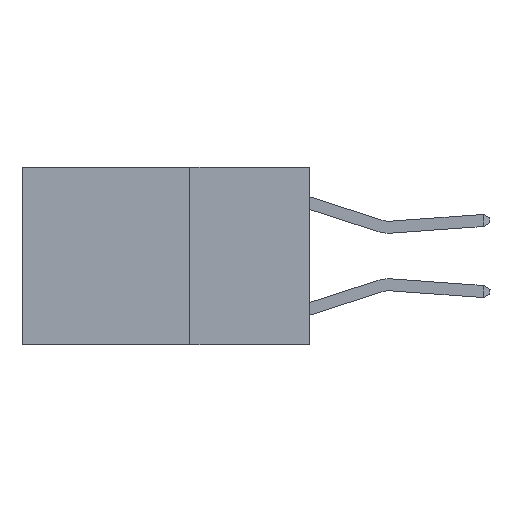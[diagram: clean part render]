
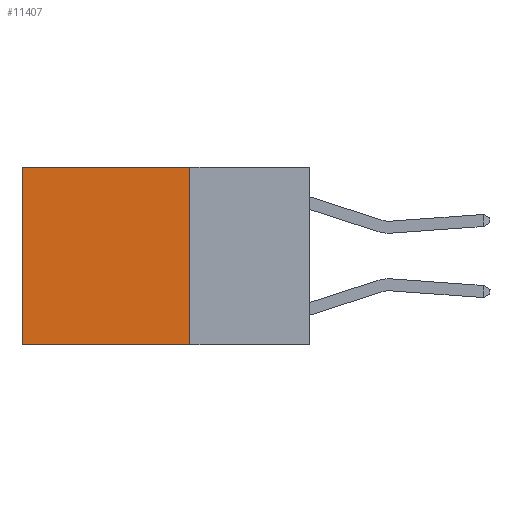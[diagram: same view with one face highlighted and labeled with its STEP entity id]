
A CAD part, left-side view. The second image highlights one B-rep face of the part: STEP entity #11407.
In plain terms, the highlighted planar face has unit normal (-1, 0, 0).
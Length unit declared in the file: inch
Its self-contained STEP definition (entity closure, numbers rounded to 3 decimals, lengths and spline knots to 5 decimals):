
#287 = CARTESIAN_POINT ( 'NONE',  ( 0.2625, 0.6, 0. ) ) ;
#1369 = DIRECTION ( 'NONE',  ( 0., 1., 0. ) ) ;
#1651 = VERTEX_POINT ( 'NONE', #30114 ) ;
#2942 = CARTESIAN_POINT ( 'NONE',  ( 0.2625, 0.25, -0.37 ) ) ;
#3785 = VECTOR ( 'NONE', #29052, 39.37008 ) ;
#3902 = DIRECTION ( 'NONE',  ( 1., 0., 0. ) ) ;
#5384 = ORIENTED_EDGE ( 'NONE', *, *, #7883, .T. ) ;
#6735 = CARTESIAN_POINT ( 'NONE',  ( 0.2625, 0.25, 0. ) ) ;
#7192 = CARTESIAN_POINT ( 'NONE',  ( 0.2625, 0.25, -0.37 ) ) ;
#7438 = VECTOR ( 'NONE', #1369, 39.37008 ) ;
#7883 = EDGE_CURVE ( 'NONE', #21939, #28550, #13767, .T. ) ;
#9365 = EDGE_LOOP ( 'NONE', ( #22935, #11660, #20960, #5384 ) ) ;
#9577 = DIRECTION ( 'NONE',  ( 0., 1., 0. ) ) ;
#11407 = ADVANCED_FACE ( 'NONE', ( #16540 ), #29983, .F. ) ;
#11660 = ORIENTED_EDGE ( 'NONE', *, *, #14592, .F. ) ;
#12200 = LINE ( 'NONE', #7192, #30407 ) ;
#12313 = DIRECTION ( 'NONE',  ( 0., 0., -1. ) ) ;
#13224 = EDGE_CURVE ( 'NONE', #21939, #27417, #22795, .T. ) ;
#13767 = LINE ( 'NONE', #29841, #7438 ) ;
#14592 = EDGE_CURVE ( 'NONE', #27417, #1651, #12200, .T. ) ;
#16540 = FACE_OUTER_BOUND ( 'NONE', #9365, .T. ) ;
#18048 = VECTOR ( 'NONE', #12313, 39.37008 ) ;
#18145 = CARTESIAN_POINT ( 'NONE',  ( 0.2625, 0.25, 0. ) ) ;
#18793 = LINE ( 'NONE', #21802, #18048 ) ;
#20551 = DIRECTION ( 'NONE',  ( 0., 0., -1. ) ) ;
#20960 = ORIENTED_EDGE ( 'NONE', *, *, #13224, .F. ) ;
#21802 = CARTESIAN_POINT ( 'NONE',  ( 0.2625, 0.6, 0. ) ) ;
#21939 = VERTEX_POINT ( 'NONE', #6735 ) ;
#22795 = LINE ( 'NONE', #26679, #3785 ) ;
#22935 = ORIENTED_EDGE ( 'NONE', *, *, #30768, .T. ) ;
#26679 = CARTESIAN_POINT ( 'NONE',  ( 0.2625, 0.25, 0. ) ) ;
#27417 = VERTEX_POINT ( 'NONE', #2942 ) ;
#28550 = VERTEX_POINT ( 'NONE', #287 ) ;
#29052 = DIRECTION ( 'NONE',  ( 0., 0., -1. ) ) ;
#29841 = CARTESIAN_POINT ( 'NONE',  ( 0.2625, 0.25, 0. ) ) ;
#29983 = PLANE ( 'NONE',  #30336 ) ;
#30114 = CARTESIAN_POINT ( 'NONE',  ( 0.2625, 0.6, -0.37 ) ) ;
#30336 = AXIS2_PLACEMENT_3D ( 'NONE', #18145, #3902, #20551 ) ;
#30407 = VECTOR ( 'NONE', #9577, 39.37008 ) ;
#30768 = EDGE_CURVE ( 'NONE', #28550, #1651, #18793, .T. ) ;
